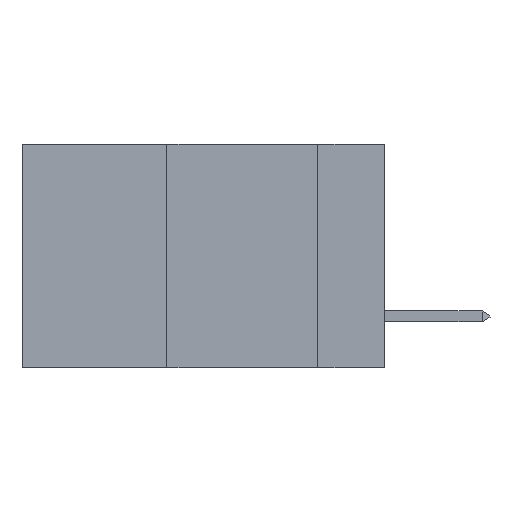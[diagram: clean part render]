
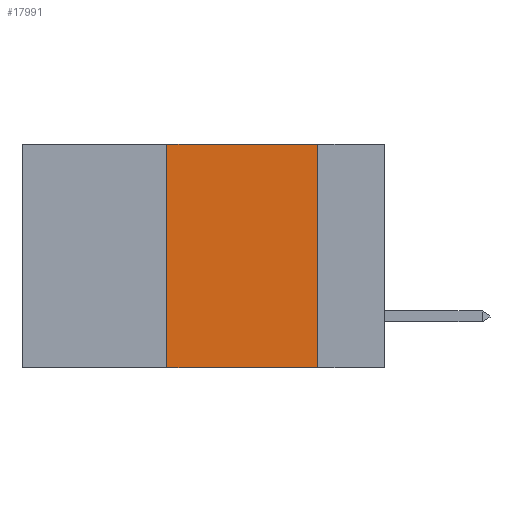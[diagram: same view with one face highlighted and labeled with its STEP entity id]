
A CAD part, left-side view. The second image highlights one B-rep face of the part: STEP entity #17991.
In plain terms, the highlighted planar face has unit normal (-1, 0, 0).
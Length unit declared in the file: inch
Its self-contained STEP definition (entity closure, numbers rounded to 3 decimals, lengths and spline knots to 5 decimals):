
#410 = DIRECTION ( 'NONE',  ( 1., 0., 0. ) ) ;
#2048 = EDGE_LOOP ( 'NONE', ( #8871, #4334, #27889, #17582 ) ) ;
#3968 = LINE ( 'NONE', #18852, #5382 ) ;
#4146 = LINE ( 'NONE', #4908, #9373 ) ;
#4334 = ORIENTED_EDGE ( 'NONE', *, *, #21169, .F. ) ;
#4516 = VECTOR ( 'NONE', #25186, 39.37008 ) ;
#4793 = AXIS2_PLACEMENT_3D ( 'NONE', #11543, #410, #16031 ) ;
#4908 = CARTESIAN_POINT ( 'NONE',  ( 0., 0.6, -0.37 ) ) ;
#5080 = CARTESIAN_POINT ( 'NONE',  ( 0., 0.36, 0. ) ) ;
#5382 = VECTOR ( 'NONE', #5536, 39.37008 ) ;
#5536 = DIRECTION ( 'NONE',  ( 0., 0., -1. ) ) ;
#6114 = CARTESIAN_POINT ( 'NONE',  ( 0., 0.6, 0. ) ) ;
#7488 = EDGE_CURVE ( 'NONE', #12341, #24977, #28075, .T. ) ;
#7626 = LINE ( 'NONE', #6114, #18719 ) ;
#8359 = DIRECTION ( 'NONE',  ( 0., -1., 0. ) ) ;
#8871 = ORIENTED_EDGE ( 'NONE', *, *, #11635, .F. ) ;
#9373 = VECTOR ( 'NONE', #27092, 39.37008 ) ;
#9576 = VERTEX_POINT ( 'NONE', #17800 ) ;
#10287 = CARTESIAN_POINT ( 'NONE',  ( 0., 0.11, -0.37 ) ) ;
#11543 = CARTESIAN_POINT ( 'NONE',  ( 0., 0.6, 0. ) ) ;
#11635 = EDGE_CURVE ( 'NONE', #9576, #11750, #3968, .T. ) ;
#11750 = VERTEX_POINT ( 'NONE', #10287 ) ;
#12341 = VERTEX_POINT ( 'NONE', #20126 ) ;
#16031 = DIRECTION ( 'NONE',  ( 0., 0., -1. ) ) ;
#16480 = CARTESIAN_POINT ( 'NONE',  ( 0., 0.36, 0. ) ) ;
#17582 = ORIENTED_EDGE ( 'NONE', *, *, #20480, .T. ) ;
#17800 = CARTESIAN_POINT ( 'NONE',  ( 0., 0.11, 0. ) ) ;
#17991 = ADVANCED_FACE ( 'NONE', ( #20972 ), #24850, .F. ) ;
#18719 = VECTOR ( 'NONE', #8359, 39.37008 ) ;
#18852 = CARTESIAN_POINT ( 'NONE',  ( 0., 0.11, 0. ) ) ;
#20126 = CARTESIAN_POINT ( 'NONE',  ( 0., 0.36, -0.37 ) ) ;
#20480 = EDGE_CURVE ( 'NONE', #12341, #11750, #4146, .T. ) ;
#20972 = FACE_OUTER_BOUND ( 'NONE', #2048, .T. ) ;
#21169 = EDGE_CURVE ( 'NONE', #24977, #9576, #7626, .T. ) ;
#24850 = PLANE ( 'NONE',  #4793 ) ;
#24977 = VERTEX_POINT ( 'NONE', #16480 ) ;
#25186 = DIRECTION ( 'NONE',  ( 0., 0., 1. ) ) ;
#27092 = DIRECTION ( 'NONE',  ( 0., -1., 0. ) ) ;
#27889 = ORIENTED_EDGE ( 'NONE', *, *, #7488, .F. ) ;
#28075 = LINE ( 'NONE', #5080, #4516 ) ;
